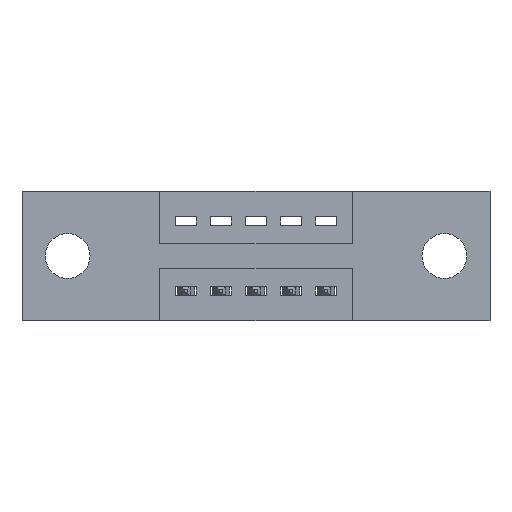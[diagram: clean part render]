
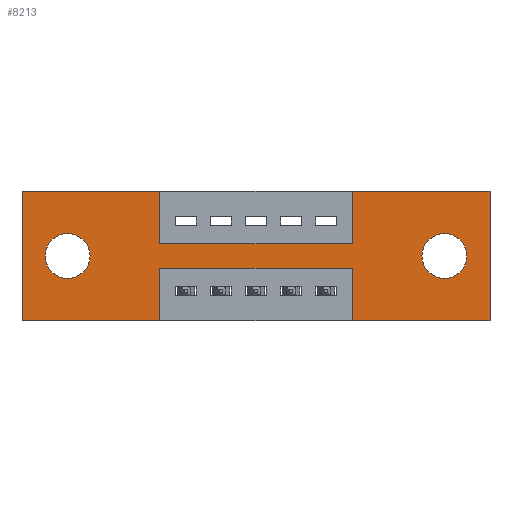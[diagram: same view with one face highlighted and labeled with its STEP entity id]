
A CAD part, front view. The second image highlights one B-rep face of the part: STEP entity #8213.
In plain terms, the highlighted planar face has unit normal (0, -1, 0).
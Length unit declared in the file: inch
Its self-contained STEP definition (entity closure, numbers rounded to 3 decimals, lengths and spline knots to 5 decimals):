
#37 = VECTOR ( 'NONE', #7891, 39.37008 ) ;
#72 = VECTOR ( 'NONE', #6194, 39.37008 ) ;
#270 = EDGE_CURVE ( 'NONE', #6035, #4398, #4003, .T. ) ;
#369 = LINE ( 'NONE', #5253, #4941 ) ;
#397 = ORIENTED_EDGE ( 'NONE', *, *, #4911, .T. ) ;
#445 = VERTEX_POINT ( 'NONE', #5291 ) ;
#468 = VERTEX_POINT ( 'NONE', #8727 ) ;
#504 = DIRECTION ( 'NONE',  ( 1., 0., 0. ) ) ;
#579 = VECTOR ( 'NONE', #6355, 39.37008 ) ;
#633 = EDGE_LOOP ( 'NONE', ( #6131, #2232, #3622, #2729, #1310, #7241, #2588, #2740, #8163, #5053, #1014, #7971 ) ) ;
#691 = VERTEX_POINT ( 'NONE', #7688 ) ;
#699 = LINE ( 'NONE', #5635, #5287 ) ;
#755 = DIRECTION ( 'NONE',  ( 0., 0., 1. ) ) ;
#905 = LINE ( 'NONE', #6985, #8114 ) ;
#942 = EDGE_CURVE ( 'NONE', #4345, #468, #5071, .T. ) ;
#945 = VERTEX_POINT ( 'NONE', #2991 ) ;
#1014 = ORIENTED_EDGE ( 'NONE', *, *, #5965, .F. ) ;
#1027 = EDGE_CURVE ( 'NONE', #5999, #3491, #8352, .T. ) ;
#1167 = AXIS2_PLACEMENT_3D ( 'NONE', #5706, #7764, #3577 ) ;
#1202 = VERTEX_POINT ( 'NONE', #6124 ) ;
#1310 = ORIENTED_EDGE ( 'NONE', *, *, #942, .F. ) ;
#1396 = EDGE_CURVE ( 'NONE', #445, #3849, #5177, .T. ) ;
#1457 = CIRCLE ( 'NONE', #4058, 0.064 ) ;
#1535 = DIRECTION ( 'NONE',  ( 0., 0., -1. ) ) ;
#1560 = CARTESIAN_POINT ( 'NONE',  ( 0.9425, 0., -0.22 ) ) ;
#1615 = AXIS2_PLACEMENT_3D ( 'NONE', #6649, #3324, #8145 ) ;
#1833 = LINE ( 'NONE', #3825, #6431 ) ;
#1865 = CARTESIAN_POINT ( 'NONE',  ( 1.205, 0., -0.249 ) ) ;
#1913 = FACE_OUTER_BOUND ( 'NONE', #633, .T. ) ;
#2045 = DIRECTION ( 'NONE',  ( 0., -1., 0. ) ) ;
#2142 = LINE ( 'NONE', #7860, #37 ) ;
#2179 = EDGE_CURVE ( 'NONE', #3491, #5999, #5488, .T. ) ;
#2195 = DIRECTION ( 'NONE',  ( 0., 1., 0. ) ) ;
#2232 = ORIENTED_EDGE ( 'NONE', *, *, #6045, .F. ) ;
#2473 = CARTESIAN_POINT ( 'NONE',  ( 0.13, 0., -0.121 ) ) ;
#2511 = CARTESIAN_POINT ( 'NONE',  ( 1.335, 0., 0. ) ) ;
#2588 = ORIENTED_EDGE ( 'NONE', *, *, #1396, .F. ) ;
#2672 = CARTESIAN_POINT ( 'NONE',  ( 0., 0., -0.37 ) ) ;
#2713 = LINE ( 'NONE', #6719, #7282 ) ;
#2729 = ORIENTED_EDGE ( 'NONE', *, *, #7021, .F. ) ;
#2740 = ORIENTED_EDGE ( 'NONE', *, *, #6888, .F. ) ;
#2900 = CARTESIAN_POINT ( 'NONE',  ( 0.13, 0., -0.185 ) ) ;
#2991 = CARTESIAN_POINT ( 'NONE',  ( 0.9425, 0., -0.37 ) ) ;
#3037 = EDGE_LOOP ( 'NONE', ( #397, #7691 ) ) ;
#3190 = CARTESIAN_POINT ( 'NONE',  ( 1.205, 0., -0.121 ) ) ;
#3324 = DIRECTION ( 'NONE',  ( 0., 1., 0. ) ) ;
#3491 = VERTEX_POINT ( 'NONE', #3190 ) ;
#3577 = DIRECTION ( 'NONE',  ( 0., 0., 1. ) ) ;
#3622 = ORIENTED_EDGE ( 'NONE', *, *, #5959, .F. ) ;
#3703 = CARTESIAN_POINT ( 'NONE',  ( 0.9425, 0., 0. ) ) ;
#3735 = CARTESIAN_POINT ( 'NONE',  ( 0., 0., -0.37 ) ) ;
#3825 = CARTESIAN_POINT ( 'NONE',  ( 0., 0., -0.37 ) ) ;
#3849 = VERTEX_POINT ( 'NONE', #3703 ) ;
#3922 = DIRECTION ( 'NONE',  ( -1., 0., 0. ) ) ;
#3946 = FACE_BOUND ( 'NONE', #3037, .T. ) ;
#4003 = CIRCLE ( 'NONE', #1167, 0.064 ) ;
#4058 = AXIS2_PLACEMENT_3D ( 'NONE', #2900, #6891, #5082 ) ;
#4110 = VECTOR ( 'NONE', #7332, 39.37008 ) ;
#4138 = PLANE ( 'NONE',  #7715 ) ;
#4257 = EDGE_CURVE ( 'NONE', #691, #8751, #8067, .T. ) ;
#4265 = CARTESIAN_POINT ( 'NONE',  ( 0.9425, 0., 0. ) ) ;
#4345 = VERTEX_POINT ( 'NONE', #2511 ) ;
#4361 = LINE ( 'NONE', #5041, #5541 ) ;
#4398 = VERTEX_POINT ( 'NONE', #2473 ) ;
#4462 = AXIS2_PLACEMENT_3D ( 'NONE', #7509, #2195, #8265 ) ;
#4557 = ORIENTED_EDGE ( 'NONE', *, *, #1027, .T. ) ;
#4668 = EDGE_CURVE ( 'NONE', #1202, #6822, #4361, .T. ) ;
#4911 = EDGE_CURVE ( 'NONE', #4398, #6035, #1457, .T. ) ;
#4941 = VECTOR ( 'NONE', #504, 39.37008 ) ;
#5041 = CARTESIAN_POINT ( 'NONE',  ( 0., 0., -0.37 ) ) ;
#5053 = ORIENTED_EDGE ( 'NONE', *, *, #4257, .F. ) ;
#5071 = LINE ( 'NONE', #8715, #579 ) ;
#5072 = LINE ( 'NONE', #6667, #4110 ) ;
#5082 = DIRECTION ( 'NONE',  ( 0., 0., 1. ) ) ;
#5177 = LINE ( 'NONE', #4265, #7585 ) ;
#5253 = CARTESIAN_POINT ( 'NONE',  ( 0.3925, 0., -0.15 ) ) ;
#5287 = VECTOR ( 'NONE', #1535, 39.37008 ) ;
#5291 = CARTESIAN_POINT ( 'NONE',  ( 0.9425, 0., -0.15 ) ) ;
#5320 = CARTESIAN_POINT ( 'NONE',  ( 0., 0., 0. ) ) ;
#5471 = CARTESIAN_POINT ( 'NONE',  ( 0.9425, 0., -0.37 ) ) ;
#5488 = CIRCLE ( 'NONE', #4462, 0.064 ) ;
#5511 = CARTESIAN_POINT ( 'NONE',  ( 0.3925, 0., 0. ) ) ;
#5517 = DIRECTION ( 'NONE',  ( 0., 0., -1. ) ) ;
#5541 = VECTOR ( 'NONE', #5726, 39.37008 ) ;
#5635 = CARTESIAN_POINT ( 'NONE',  ( 0.3925, 0., 0. ) ) ;
#5706 = CARTESIAN_POINT ( 'NONE',  ( 0.13, 0., -0.185 ) ) ;
#5726 = DIRECTION ( 'NONE',  ( -1., 0., 0. ) ) ;
#5865 = VERTEX_POINT ( 'NONE', #7915 ) ;
#5905 = DIRECTION ( 'NONE',  ( -1., 0., 0. ) ) ;
#5959 = EDGE_CURVE ( 'NONE', #945, #7294, #7931, .T. ) ;
#5965 = EDGE_CURVE ( 'NONE', #6822, #691, #5072, .T. ) ;
#5999 = VERTEX_POINT ( 'NONE', #1865 ) ;
#6035 = VERTEX_POINT ( 'NONE', #7302 ) ;
#6045 = EDGE_CURVE ( 'NONE', #7294, #8675, #2713, .T. ) ;
#6124 = CARTESIAN_POINT ( 'NONE',  ( 0.3925, 0., -0.37 ) ) ;
#6131 = ORIENTED_EDGE ( 'NONE', *, *, #6744, .F. ) ;
#6194 = DIRECTION ( 'NONE',  ( 0., 0., 1. ) ) ;
#6211 = EDGE_CURVE ( 'NONE', #8751, #5865, #699, .T. ) ;
#6355 = DIRECTION ( 'NONE',  ( 0., 0., -1. ) ) ;
#6405 = DIRECTION ( 'NONE',  ( 0., 0., -1. ) ) ;
#6415 = DIRECTION ( 'NONE',  ( 1., 0., 0. ) ) ;
#6431 = VECTOR ( 'NONE', #5905, 39.37008 ) ;
#6594 = VECTOR ( 'NONE', #6415, 39.37008 ) ;
#6649 = CARTESIAN_POINT ( 'NONE',  ( 1.205, 0., -0.185 ) ) ;
#6667 = CARTESIAN_POINT ( 'NONE',  ( 0., 0., 0. ) ) ;
#6719 = CARTESIAN_POINT ( 'NONE',  ( 0.3925, 0., -0.22 ) ) ;
#6744 = EDGE_CURVE ( 'NONE', #8675, #1202, #905, .T. ) ;
#6822 = VERTEX_POINT ( 'NONE', #3735 ) ;
#6888 = EDGE_CURVE ( 'NONE', #5865, #445, #369, .T. ) ;
#6891 = DIRECTION ( 'NONE',  ( 0., 1., 0. ) ) ;
#6985 = CARTESIAN_POINT ( 'NONE',  ( 0.3925, 0., -0.37 ) ) ;
#7018 = ORIENTED_EDGE ( 'NONE', *, *, #2179, .T. ) ;
#7021 = EDGE_CURVE ( 'NONE', #468, #945, #1833, .T. ) ;
#7241 = ORIENTED_EDGE ( 'NONE', *, *, #7538, .F. ) ;
#7282 = VECTOR ( 'NONE', #3922, 39.37008 ) ;
#7294 = VERTEX_POINT ( 'NONE', #1560 ) ;
#7302 = CARTESIAN_POINT ( 'NONE',  ( 0.13, 0., -0.249 ) ) ;
#7332 = DIRECTION ( 'NONE',  ( 0., 0., 1. ) ) ;
#7509 = CARTESIAN_POINT ( 'NONE',  ( 1.205, 0., -0.185 ) ) ;
#7538 = EDGE_CURVE ( 'NONE', #3849, #4345, #2142, .T. ) ;
#7585 = VECTOR ( 'NONE', #755, 39.37008 ) ;
#7688 = CARTESIAN_POINT ( 'NONE',  ( 0., 0., 0. ) ) ;
#7691 = ORIENTED_EDGE ( 'NONE', *, *, #270, .T. ) ;
#7715 = AXIS2_PLACEMENT_3D ( 'NONE', #2672, #2045, #5517 ) ;
#7764 = DIRECTION ( 'NONE',  ( 0., 1., 0. ) ) ;
#7860 = CARTESIAN_POINT ( 'NONE',  ( 0., 0., 0. ) ) ;
#7891 = DIRECTION ( 'NONE',  ( 1., 0., 0. ) ) ;
#7915 = CARTESIAN_POINT ( 'NONE',  ( 0.3925, 0., -0.15 ) ) ;
#7931 = LINE ( 'NONE', #5471, #72 ) ;
#7934 = EDGE_LOOP ( 'NONE', ( #7018, #4557 ) ) ;
#7971 = ORIENTED_EDGE ( 'NONE', *, *, #4668, .F. ) ;
#7991 = FACE_BOUND ( 'NONE', #7934, .T. ) ;
#8067 = LINE ( 'NONE', #5320, #6594 ) ;
#8114 = VECTOR ( 'NONE', #6405, 39.37008 ) ;
#8145 = DIRECTION ( 'NONE',  ( 0., 0., -1. ) ) ;
#8163 = ORIENTED_EDGE ( 'NONE', *, *, #6211, .F. ) ;
#8213 = ADVANCED_FACE ( 'NONE', ( #7991, #3946, #1913 ), #4138, .T. ) ;
#8265 = DIRECTION ( 'NONE',  ( 0., 0., -1. ) ) ;
#8352 = CIRCLE ( 'NONE', #1615, 0.064 ) ;
#8532 = CARTESIAN_POINT ( 'NONE',  ( 0.3925, 0., -0.22 ) ) ;
#8675 = VERTEX_POINT ( 'NONE', #8532 ) ;
#8715 = CARTESIAN_POINT ( 'NONE',  ( 1.335, 0., 0. ) ) ;
#8727 = CARTESIAN_POINT ( 'NONE',  ( 1.335, 0., -0.37 ) ) ;
#8751 = VERTEX_POINT ( 'NONE', #5511 ) ;
